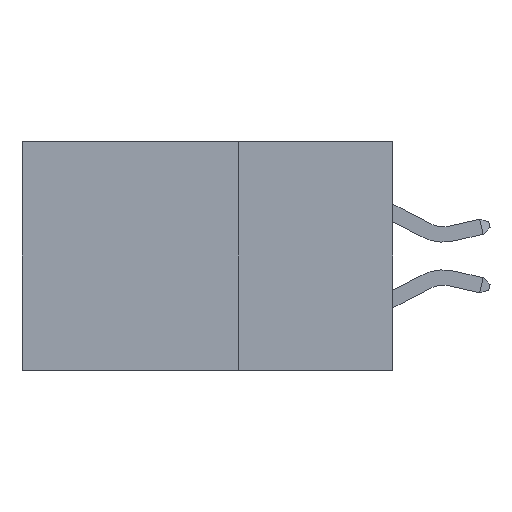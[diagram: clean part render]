
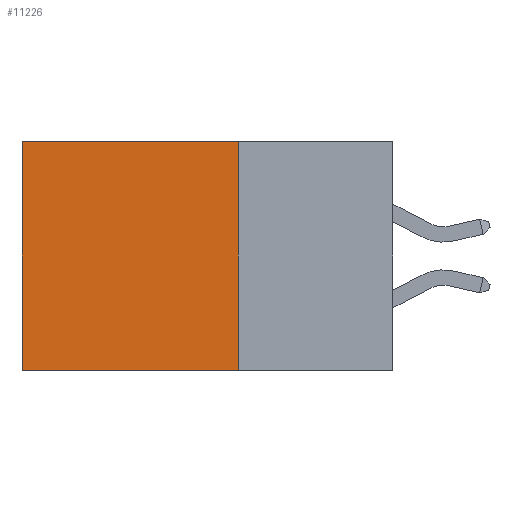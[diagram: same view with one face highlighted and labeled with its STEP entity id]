
A CAD part, left-side view. The second image highlights one B-rep face of the part: STEP entity #11226.
In plain terms, the highlighted planar face has unit normal (-1, 0, 0).
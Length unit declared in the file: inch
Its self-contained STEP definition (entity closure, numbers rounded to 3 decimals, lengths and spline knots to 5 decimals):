
#799 = EDGE_CURVE ( 'NONE', #2862, #22676, #20867, .T. ) ;
#932 = VECTOR ( 'NONE', #23205, 39.37008 ) ;
#2586 = VERTEX_POINT ( 'NONE', #36770 ) ;
#2862 = VERTEX_POINT ( 'NONE', #29077 ) ;
#3499 = ORIENTED_EDGE ( 'NONE', *, *, #16547, .T. ) ;
#4769 = CARTESIAN_POINT ( 'NONE',  ( 0.2875, 0.25, 0. ) ) ;
#5444 = DIRECTION ( 'NONE',  ( 0., 0., -1. ) ) ;
#5468 = CARTESIAN_POINT ( 'NONE',  ( 0.2875, 0.6, 0. ) ) ;
#6285 = VECTOR ( 'NONE', #26421, 39.37008 ) ;
#6888 = EDGE_CURVE ( 'NONE', #2586, #2862, #38675, .T. ) ;
#8101 = FACE_OUTER_BOUND ( 'NONE', #19085, .T. ) ;
#8236 = ORIENTED_EDGE ( 'NONE', *, *, #799, .F. ) ;
#10798 = CARTESIAN_POINT ( 'NONE',  ( 0.2875, 0.6, 0. ) ) ;
#11226 = ADVANCED_FACE ( 'NONE', ( #8101 ), #38531, .F. ) ;
#12877 = DIRECTION ( 'NONE',  ( 0., 1., 0. ) ) ;
#13776 = LINE ( 'NONE', #10798, #6285 ) ;
#14171 = VECTOR ( 'NONE', #36018, 39.37008 ) ;
#16547 = EDGE_CURVE ( 'NONE', #23410, #22676, #13776, .T. ) ;
#16722 = LINE ( 'NONE', #30995, #33754 ) ;
#19085 = EDGE_LOOP ( 'NONE', ( #3499, #8236, #20468, #35410 ) ) ;
#20468 = ORIENTED_EDGE ( 'NONE', *, *, #6888, .F. ) ;
#20867 = LINE ( 'NONE', #33078, #14171 ) ;
#22676 = VERTEX_POINT ( 'NONE', #25786 ) ;
#23205 = DIRECTION ( 'NONE',  ( 0., 0., -1. ) ) ;
#23410 = VERTEX_POINT ( 'NONE', #5468 ) ;
#25301 = AXIS2_PLACEMENT_3D ( 'NONE', #32550, #29816, #5444 ) ;
#25786 = CARTESIAN_POINT ( 'NONE',  ( 0.2875, 0.6, -0.37 ) ) ;
#26421 = DIRECTION ( 'NONE',  ( 0., 0., -1. ) ) ;
#29077 = CARTESIAN_POINT ( 'NONE',  ( 0.2875, 0.25, -0.37 ) ) ;
#29816 = DIRECTION ( 'NONE',  ( 1., 0., 0. ) ) ;
#30316 = EDGE_CURVE ( 'NONE', #2586, #23410, #16722, .T. ) ;
#30995 = CARTESIAN_POINT ( 'NONE',  ( 0.2875, 0.25, 0. ) ) ;
#32550 = CARTESIAN_POINT ( 'NONE',  ( 0.2875, 0.25, 0. ) ) ;
#33078 = CARTESIAN_POINT ( 'NONE',  ( 0.2875, 0.25, -0.37 ) ) ;
#33754 = VECTOR ( 'NONE', #12877, 39.37008 ) ;
#35410 = ORIENTED_EDGE ( 'NONE', *, *, #30316, .T. ) ;
#36018 = DIRECTION ( 'NONE',  ( 0., 1., 0. ) ) ;
#36770 = CARTESIAN_POINT ( 'NONE',  ( 0.2875, 0.25, 0. ) ) ;
#38531 = PLANE ( 'NONE',  #25301 ) ;
#38675 = LINE ( 'NONE', #4769, #932 ) ;
